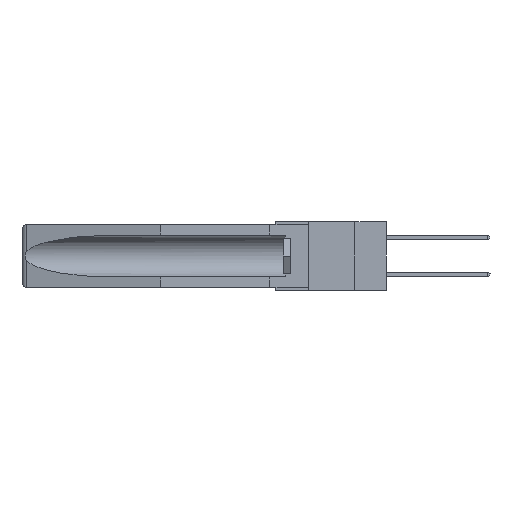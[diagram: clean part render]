
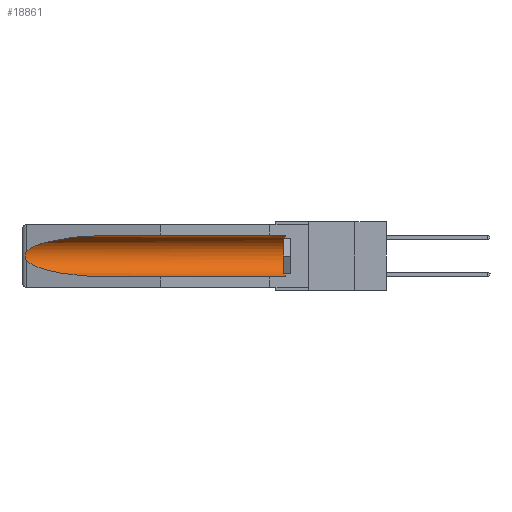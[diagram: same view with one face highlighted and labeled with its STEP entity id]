
A CAD part, left-side view. The second image highlights one B-rep face of the part: STEP entity #18861.
In plain terms, the highlighted cylindrical face has radius 2.857 mm (diameter 5.715 mm), a partial arc.
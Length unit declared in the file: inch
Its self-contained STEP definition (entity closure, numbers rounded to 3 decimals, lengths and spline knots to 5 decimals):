
#1521 = LINE ( 'NONE', #2319, #4786 ) ;
#2264 = EDGE_CURVE ( 'NONE', #16837, #10011, #21607, .T. ) ;
#2319 = CARTESIAN_POINT ( 'NONE',  ( 0.155, -0.30754, -0.284 ) ) ;
#2423 = DIRECTION ( 'NONE',  ( 0., 1., 0. ) ) ;
#2513 = CARTESIAN_POINT ( 'NONE',  ( 0.2675, 1.53308, -0.17534 ) ) ;
#2612 = CARTESIAN_POINT ( 'NONE',  ( 0.2673, 1.53269, -0.17917 ) ) ;
#2622 = ORIENTED_EDGE ( 'NONE', *, *, #15161, .T. ) ;
#2918 = VECTOR ( 'NONE', #11849, 39.37008 ) ;
#4268 = EDGE_CURVE ( 'NONE', #20838, #21526, #21920, .T. ) ;
#4786 = VECTOR ( 'NONE', #2423, 39.37008 ) ;
#6807 = CYLINDRICAL_SURFACE ( 'NONE', #27672, 0.1125 ) ;
#7022 = EDGE_CURVE ( 'NONE', #21526, #29789, #11023, .T. ) ;
#7323 = CARTESIAN_POINT ( 'NONE',  ( 0.26537, 1.52718, -0.19328 ) ) ;
#7948 = ORIENTED_EDGE ( 'NONE', *, *, #19168, .T. ) ;
#9068 =( BOUNDED_CURVE ( )  B_SPLINE_CURVE ( 3, ( #22249, #12831, #17590, #19957 ),
 .UNSPECIFIED., .F., .F. ) 
 B_SPLINE_CURVE_WITH_KNOTS ( ( 4, 4 ),
 ( 4.71239, 6.08839 ),
 .UNSPECIFIED. ) 
 CURVE ( )  GEOMETRIC_REPRESENTATION_ITEM ( )  RATIONAL_B_SPLINE_CURVE ( ( 1., 0.848, 0.848, 1. ) ) 
 REPRESENTATION_ITEM ( '' )  );
#9609 = CARTESIAN_POINT ( 'NONE',  ( 0.26537, 1.52718, -0.14972 ) ) ;
#10011 = VERTEX_POINT ( 'NONE', #20619 ) ;
#11023 = LINE ( 'NONE', #19097, #2918 ) ;
#11837 = CARTESIAN_POINT ( 'NONE',  ( 0.155, 1.07973, -0.059 ) ) ;
#11849 = DIRECTION ( 'NONE',  ( 0., 1., 0. ) ) ;
#12831 = CARTESIAN_POINT ( 'NONE',  ( 0.21114, 1.30732, -0.059 ) ) ;
#13429 = ORIENTED_EDGE ( 'NONE', *, *, #4268, .T. ) ;
#13571 = CARTESIAN_POINT ( 'NONE',  ( 0.26537, 1.52718, -0.19328 ) ) ;
#13739 = ORIENTED_EDGE ( 'NONE', *, *, #2264, .T. ) ;
#14108 = AXIS2_PLACEMENT_3D ( 'NONE', #18891, #30631, #21384 ) ;
#15161 = EDGE_CURVE ( 'NONE', #25452, #16837, #24835, .T. ) ;
#16655 = CARTESIAN_POINT ( 'NONE',  ( 0.155, -0.30754, -0.1715 ) ) ;
#16759 = CARTESIAN_POINT ( 'NONE',  ( 0.26655, 1.53094, -0.18657 ) ) ;
#16837 = VERTEX_POINT ( 'NONE', #13571 ) ;
#17192 = EDGE_LOOP ( 'NONE', ( #7948, #2622, #13739, #24324, #13429, #18600 ) ) ;
#17590 = CARTESIAN_POINT ( 'NONE',  ( 0.25451, 1.48313, -0.09465 ) ) ;
#18248 = CARTESIAN_POINT ( 'NONE',  ( 0.155, 0.126, -0.059 ) ) ;
#18600 = ORIENTED_EDGE ( 'NONE', *, *, #7022, .T. ) ;
#18728 = DIRECTION ( 'NONE',  ( 0., 1., 0. ) ) ;
#18861 = ADVANCED_FACE ( 'NONE', ( #25711 ), #6807, .F. ) ;
#18891 = CARTESIAN_POINT ( 'NONE',  ( 0.155, 0.126, -0.1715 ) ) ;
#18940 = CARTESIAN_POINT ( 'NONE',  ( 0.26654, 1.53092, -0.15636 ) ) ;
#19035 = DIRECTION ( 'NONE',  ( 0., 0., 1. ) ) ;
#19039 = CARTESIAN_POINT ( 'NONE',  ( 0.2673, 1.5327, -0.16383 ) ) ;
#19097 = CARTESIAN_POINT ( 'NONE',  ( 0.155, -0.30754, -0.059 ) ) ;
#19168 = EDGE_CURVE ( 'NONE', #29789, #25452, #9068, .T. ) ;
#19957 = CARTESIAN_POINT ( 'NONE',  ( 0.26537, 1.52718, -0.14972 ) ) ;
#20619 = CARTESIAN_POINT ( 'NONE',  ( 0.155, 1.07973, -0.284 ) ) ;
#20770 = CARTESIAN_POINT ( 'NONE',  ( 0.26537, 1.52718, -0.19328 ) ) ;
#20838 = VERTEX_POINT ( 'NONE', #24394 ) ;
#21384 = DIRECTION ( 'NONE',  ( 0., 0., 1. ) ) ;
#21436 = CARTESIAN_POINT ( 'NONE',  ( 0.2675, 1.53308, -0.16763 ) ) ;
#21526 = VERTEX_POINT ( 'NONE', #18248 ) ;
#21539 = CARTESIAN_POINT ( 'NONE',  ( 0.26597, 1.5296, -0.19026 ) ) ;
#21607 =( BOUNDED_CURVE ( )  B_SPLINE_CURVE ( 3, ( #20770, #30431, #23155, #28124 ),
 .UNSPECIFIED., .F., .F. ) 
 B_SPLINE_CURVE_WITH_KNOTS ( ( 4, 4 ),
 ( 0.1948, 1.5708 ),
 .UNSPECIFIED. ) 
 CURVE ( )  GEOMETRIC_REPRESENTATION_ITEM ( )  RATIONAL_B_SPLINE_CURVE ( ( 1., 0.848, 0.848, 1. ) ) 
 REPRESENTATION_ITEM ( '' )  );
#21766 = EDGE_CURVE ( 'NONE', #20838, #10011, #1521, .T. ) ;
#21920 = CIRCLE ( 'NONE', #14108, 0.1125 ) ;
#22249 = CARTESIAN_POINT ( 'NONE',  ( 0.155, 1.07973, -0.059 ) ) ;
#23155 = CARTESIAN_POINT ( 'NONE',  ( 0.21114, 1.30732, -0.284 ) ) ;
#24324 = ORIENTED_EDGE ( 'NONE', *, *, #21766, .F. ) ;
#24394 = CARTESIAN_POINT ( 'NONE',  ( 0.155, 0.126, -0.284 ) ) ;
#24835 = B_SPLINE_CURVE_WITH_KNOTS ( 'NONE', 3,
 ( #9609, #28481, #18940, #19039, #21436, #2513, #2612, #16759, #21539, #7323 ),
 .UNSPECIFIED., .F., .F.,
 ( 4, 2, 2, 2, 4 ),
 ( 0., 0.00029, 0.00058, 0.00087, 0.00117 ),
 .UNSPECIFIED. ) ;
#25452 = VERTEX_POINT ( 'NONE', #30655 ) ;
#25711 = FACE_OUTER_BOUND ( 'NONE', #17192, .T. ) ;
#27672 = AXIS2_PLACEMENT_3D ( 'NONE', #16655, #18728, #19035 ) ;
#28124 = CARTESIAN_POINT ( 'NONE',  ( 0.155, 1.07973, -0.284 ) ) ;
#28481 = CARTESIAN_POINT ( 'NONE',  ( 0.26597, 1.52961, -0.15275 ) ) ;
#29789 = VERTEX_POINT ( 'NONE', #11837 ) ;
#30431 = CARTESIAN_POINT ( 'NONE',  ( 0.25451, 1.48313, -0.24835 ) ) ;
#30631 = DIRECTION ( 'NONE',  ( 0., -1., 0. ) ) ;
#30655 = CARTESIAN_POINT ( 'NONE',  ( 0.26537, 1.52718, -0.14972 ) ) ;
